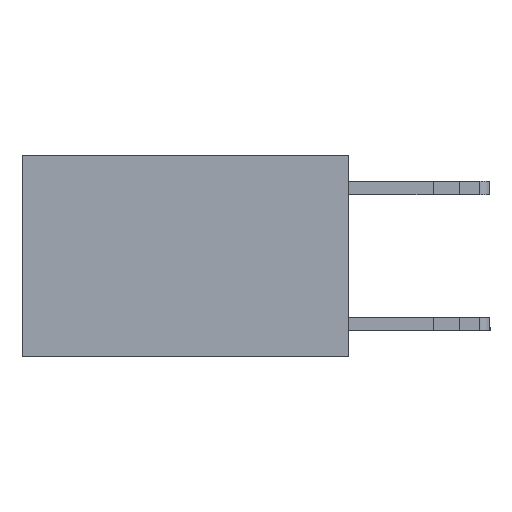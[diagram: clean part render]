
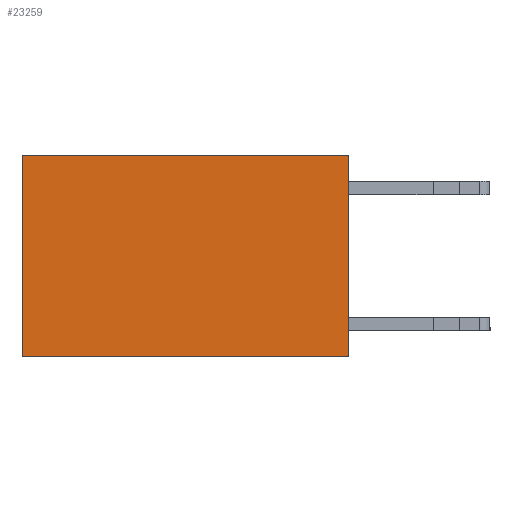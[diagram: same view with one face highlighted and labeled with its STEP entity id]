
A CAD part, left-side view. The second image highlights one B-rep face of the part: STEP entity #23259.
In plain terms, the highlighted planar face has unit normal (-1, 0, 0).
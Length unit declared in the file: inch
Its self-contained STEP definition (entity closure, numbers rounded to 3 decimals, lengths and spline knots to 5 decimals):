
#780 = LINE ( 'NONE', #6602, #22954 ) ;
#1578 = VERTEX_POINT ( 'NONE', #4620 ) ;
#1775 = CARTESIAN_POINT ( 'NONE',  ( 0.2625, 0., -0.37 ) ) ;
#2445 = CARTESIAN_POINT ( 'NONE',  ( 0.2625, 0., 0. ) ) ;
#3221 = DIRECTION ( 'NONE',  ( 0., 0., -1. ) ) ;
#4110 = CARTESIAN_POINT ( 'NONE',  ( 0.2625, 0., -0.37 ) ) ;
#4341 = LINE ( 'NONE', #9918, #18193 ) ;
#4427 = VECTOR ( 'NONE', #3221, 39.37008 ) ;
#4620 = CARTESIAN_POINT ( 'NONE',  ( 0.2625, 0., 0. ) ) ;
#6309 = LINE ( 'NONE', #4110, #20473 ) ;
#6602 = CARTESIAN_POINT ( 'NONE',  ( 0.2625, 0.6, 0. ) ) ;
#7218 = ORIENTED_EDGE ( 'NONE', *, *, #12586, .F. ) ;
#7358 = ORIENTED_EDGE ( 'NONE', *, *, #9405, .T. ) ;
#9405 = EDGE_CURVE ( 'NONE', #15714, #12985, #780, .T. ) ;
#9654 = CARTESIAN_POINT ( 'NONE',  ( 0.2625, 0.6, 0. ) ) ;
#9918 = CARTESIAN_POINT ( 'NONE',  ( 0.2625, 0., 0. ) ) ;
#10579 = DIRECTION ( 'NONE',  ( 0., 0., -1. ) ) ;
#12586 = EDGE_CURVE ( 'NONE', #1578, #18382, #22764, .T. ) ;
#12985 = VERTEX_POINT ( 'NONE', #18732 ) ;
#15714 = VERTEX_POINT ( 'NONE', #9654 ) ;
#15847 = EDGE_CURVE ( 'NONE', #1578, #15714, #4341, .T. ) ;
#15848 = DIRECTION ( 'NONE',  ( 0., 1., 0. ) ) ;
#15943 = AXIS2_PLACEMENT_3D ( 'NONE', #2445, #18366, #20186 ) ;
#18193 = VECTOR ( 'NONE', #15848, 39.37008 ) ;
#18217 = ORIENTED_EDGE ( 'NONE', *, *, #21968, .F. ) ;
#18366 = DIRECTION ( 'NONE',  ( 1., 0., 0. ) ) ;
#18382 = VERTEX_POINT ( 'NONE', #1775 ) ;
#18732 = CARTESIAN_POINT ( 'NONE',  ( 0.2625, 0.6, -0.37 ) ) ;
#20186 = DIRECTION ( 'NONE',  ( 0., 0., -1. ) ) ;
#20473 = VECTOR ( 'NONE', #22073, 39.37008 ) ;
#20573 = FACE_OUTER_BOUND ( 'NONE', #23197, .T. ) ;
#20827 = CARTESIAN_POINT ( 'NONE',  ( 0.2625, 0., 0. ) ) ;
#21968 = EDGE_CURVE ( 'NONE', #18382, #12985, #6309, .T. ) ;
#22073 = DIRECTION ( 'NONE',  ( 0., 1., 0. ) ) ;
#22764 = LINE ( 'NONE', #20827, #4427 ) ;
#22954 = VECTOR ( 'NONE', #10579, 39.37008 ) ;
#23197 = EDGE_LOOP ( 'NONE', ( #7358, #18217, #7218, #24643 ) ) ;
#23259 = ADVANCED_FACE ( 'NONE', ( #20573 ), #24321, .F. ) ;
#24321 = PLANE ( 'NONE',  #15943 ) ;
#24643 = ORIENTED_EDGE ( 'NONE', *, *, #15847, .T. ) ;
